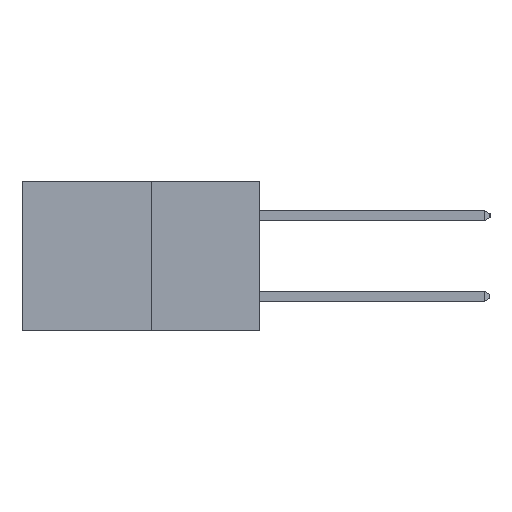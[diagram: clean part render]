
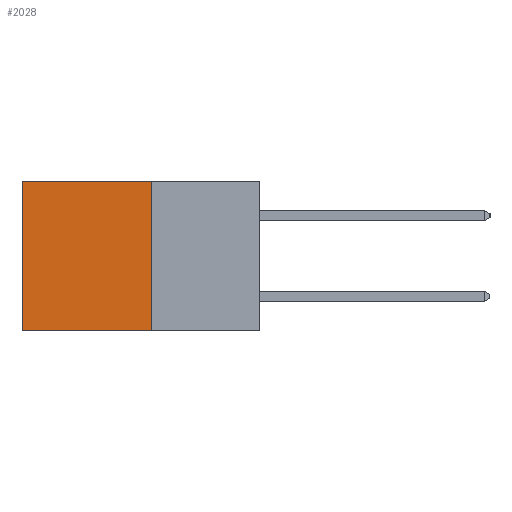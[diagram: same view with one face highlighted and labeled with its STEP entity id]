
A CAD part, left-side view. The second image highlights one B-rep face of the part: STEP entity #2028.
In plain terms, the highlighted planar face has unit normal (-1, 0, 0).
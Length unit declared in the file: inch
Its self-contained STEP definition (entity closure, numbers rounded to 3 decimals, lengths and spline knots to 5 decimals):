
#199 = ORIENTED_EDGE ( 'NONE', *, *, #932, .F. ) ;
#363 = CARTESIAN_POINT ( 'NONE',  ( 0.277, 0.27, -0.37 ) ) ;
#904 = PLANE ( 'NONE',  #6180 ) ;
#932 = EDGE_CURVE ( 'NONE', #8411, #4050, #5951, .T. ) ;
#1332 = FACE_OUTER_BOUND ( 'NONE', #4962, .T. ) ;
#1512 = ORIENTED_EDGE ( 'NONE', *, *, #8646, .F. ) ;
#2028 = ADVANCED_FACE ( 'NONE', ( #1332 ), #904, .F. ) ;
#2288 = CARTESIAN_POINT ( 'NONE',  ( 0.277, 0.27, -0.37 ) ) ;
#2770 = DIRECTION ( 'NONE',  ( 0., 0., -1. ) ) ;
#2796 = CARTESIAN_POINT ( 'NONE',  ( 0.277, 0.59, -0.37 ) ) ;
#3040 = LINE ( 'NONE', #2796, #7449 ) ;
#3087 = DIRECTION ( 'NONE',  ( 1., 0., 0. ) ) ;
#3161 = VERTEX_POINT ( 'NONE', #10869 ) ;
#3227 = DIRECTION ( 'NONE',  ( 0., 1., 0. ) ) ;
#3280 = VERTEX_POINT ( 'NONE', #9168 ) ;
#3437 = CARTESIAN_POINT ( 'NONE',  ( 0.277, 0.27, -0.37 ) ) ;
#3503 = ORIENTED_EDGE ( 'NONE', *, *, #9151, .T. ) ;
#3573 = DIRECTION ( 'NONE',  ( 0., 0., -1. ) ) ;
#3682 = DIRECTION ( 'NONE',  ( 0., 0., -1. ) ) ;
#3864 = VECTOR ( 'NONE', #8584, 39.37008 ) ;
#4009 = VECTOR ( 'NONE', #3227, 39.37008 ) ;
#4050 = VERTEX_POINT ( 'NONE', #9216 ) ;
#4189 = EDGE_CURVE ( 'NONE', #8411, #3280, #10671, .T. ) ;
#4962 = EDGE_LOOP ( 'NONE', ( #3503, #1512, #199, #5268 ) ) ;
#5268 = ORIENTED_EDGE ( 'NONE', *, *, #4189, .T. ) ;
#5951 = LINE ( 'NONE', #363, #8049 ) ;
#6180 = AXIS2_PLACEMENT_3D ( 'NONE', #3437, #3087, #3573 ) ;
#7449 = VECTOR ( 'NONE', #3682, 39.37008 ) ;
#7923 = CARTESIAN_POINT ( 'NONE',  ( 0.277, 0.27, 0. ) ) ;
#8049 = VECTOR ( 'NONE', #2770, 39.37008 ) ;
#8345 = CARTESIAN_POINT ( 'NONE',  ( 0.277, 0.27, 0. ) ) ;
#8411 = VERTEX_POINT ( 'NONE', #8345 ) ;
#8584 = DIRECTION ( 'NONE',  ( 0., 1., 0. ) ) ;
#8646 = EDGE_CURVE ( 'NONE', #4050, #3161, #10802, .T. ) ;
#9151 = EDGE_CURVE ( 'NONE', #3280, #3161, #3040, .T. ) ;
#9168 = CARTESIAN_POINT ( 'NONE',  ( 0.277, 0.59, 0. ) ) ;
#9216 = CARTESIAN_POINT ( 'NONE',  ( 0.277, 0.27, -0.37 ) ) ;
#10671 = LINE ( 'NONE', #7923, #3864 ) ;
#10802 = LINE ( 'NONE', #2288, #4009 ) ;
#10869 = CARTESIAN_POINT ( 'NONE',  ( 0.277, 0.59, -0.37 ) ) ;
